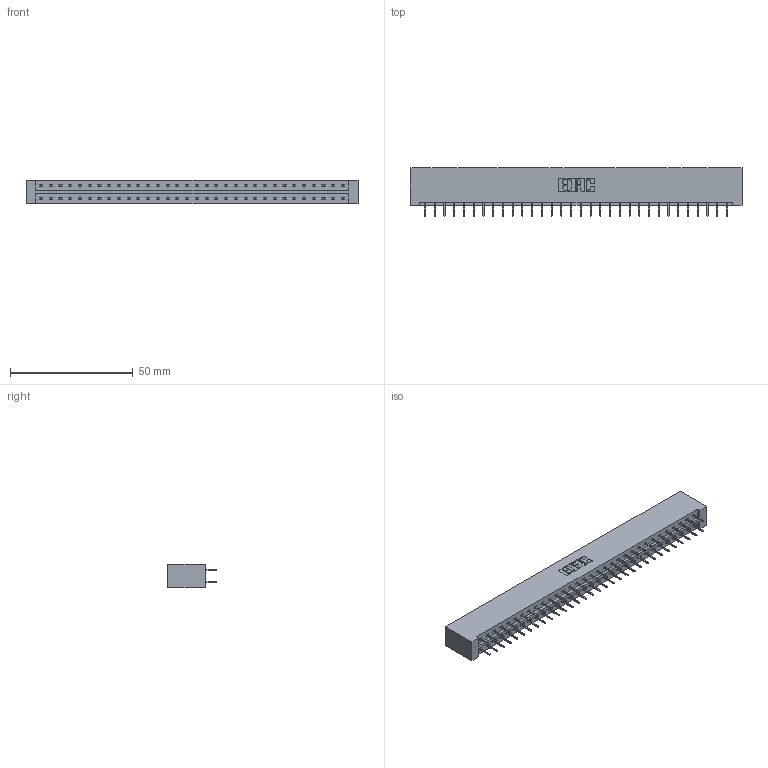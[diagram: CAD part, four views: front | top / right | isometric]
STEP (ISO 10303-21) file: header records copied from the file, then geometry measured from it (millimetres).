
FILE_DESCRIPTION (( 'STEP AP203' ), '1' );
FILE_NAME ('333-064-524-201.STEP', '2018-08-04T09:43:58', ( '' ), ( '' ), 'SwSTEP 2.0', 'SolidWorks 2016', '' );
FILE_SCHEMA (( 'CONFIG_CONTROL_DESIGN' ));
Length unit declared in the file: inch
Products named in the file (3): 333 Part_Lugless; 345-292-001_345-293-124; 333-064-524-201
Assembly tree (65 placements, depth 2):
  333-064-524-201
    333 Part_Lugless
    345-292-001_345-293-124  x64
Bounding box: 135.05 x 19.69 x 9.4 mm (x, y, z)
Volume: 14229.9 mm3; surface area: 16449.5 mm2
Topology: 65 solids, 65 shells, 3690 faces, 10463 edges, 6718 vertices
Faces by surface type: plane 2754, cylinder 936
Entity records: 21677 total; most frequent: CARTESIAN_POINT 3602, ORIENTED_EDGE 3538, DIRECTION 3089, EDGE_CURVE 1769, LINE 1653, VECTOR 1653, VERTEX_POINT 1174, AXIS2_PLACEMENT_3D 718
